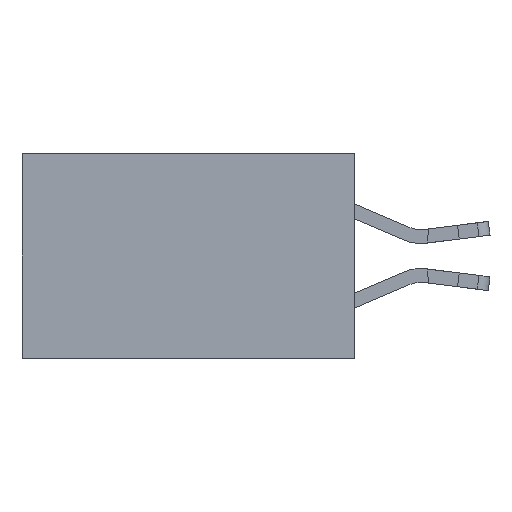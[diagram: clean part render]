
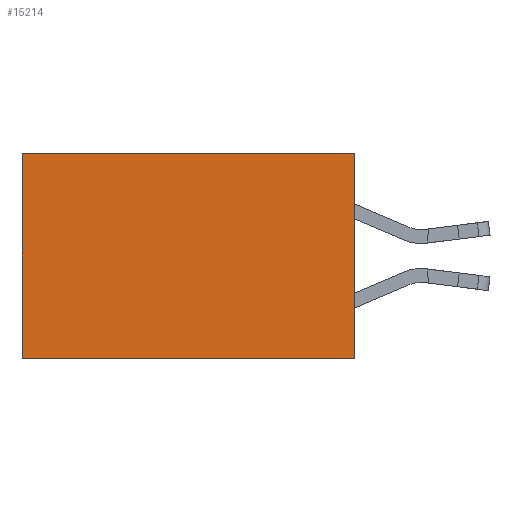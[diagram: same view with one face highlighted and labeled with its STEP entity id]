
A CAD part, left-side view. The second image highlights one B-rep face of the part: STEP entity #15214.
In plain terms, the highlighted planar face has unit normal (-1, 0, 0).
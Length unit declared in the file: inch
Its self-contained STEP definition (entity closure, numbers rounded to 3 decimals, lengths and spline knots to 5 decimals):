
#25 = CARTESIAN_POINT ( 'NONE',  ( 0.298, 0., 0. ) ) ;
#1028 = ORIENTED_EDGE ( 'NONE', *, *, #16419, .T. ) ;
#1622 = AXIS2_PLACEMENT_3D ( 'NONE', #9957, #19047, #8175 ) ;
#1727 = EDGE_CURVE ( 'NONE', #8493, #19266, #16690, .T. ) ;
#2264 = CARTESIAN_POINT ( 'NONE',  ( 0.298, 0.6, 0. ) ) ;
#2305 = CARTESIAN_POINT ( 'NONE',  ( 0.298, 0., -0.37 ) ) ;
#2420 = CARTESIAN_POINT ( 'NONE',  ( 0.298, 0., 0. ) ) ;
#2468 = PLANE ( 'NONE',  #1622 ) ;
#4187 = LINE ( 'NONE', #2420, #22851 ) ;
#4467 = DIRECTION ( 'NONE',  ( 0., 1., 0. ) ) ;
#8175 = DIRECTION ( 'NONE',  ( 0., 0., -1. ) ) ;
#8493 = VERTEX_POINT ( 'NONE', #21633 ) ;
#8758 = VERTEX_POINT ( 'NONE', #2305 ) ;
#9016 = LINE ( 'NONE', #18763, #22746 ) ;
#9944 = VECTOR ( 'NONE', #12776, 39.37008 ) ;
#9957 = CARTESIAN_POINT ( 'NONE',  ( 0.298, 0., 0. ) ) ;
#11670 = EDGE_CURVE ( 'NONE', #8493, #8758, #4187, .T. ) ;
#11804 = DIRECTION ( 'NONE',  ( 0., 0., -1. ) ) ;
#11878 = VECTOR ( 'NONE', #4467, 39.37008 ) ;
#12776 = DIRECTION ( 'NONE',  ( 0., 1., 0. ) ) ;
#14910 = EDGE_CURVE ( 'NONE', #8758, #15869, #19004, .T. ) ;
#15214 = ADVANCED_FACE ( 'NONE', ( #22249 ), #2468, .F. ) ;
#15481 = ORIENTED_EDGE ( 'NONE', *, *, #1727, .T. ) ;
#15865 = ORIENTED_EDGE ( 'NONE', *, *, #14910, .F. ) ;
#15869 = VERTEX_POINT ( 'NONE', #22524 ) ;
#16419 = EDGE_CURVE ( 'NONE', #19266, #15869, #9016, .T. ) ;
#16690 = LINE ( 'NONE', #25, #11878 ) ;
#17492 = ORIENTED_EDGE ( 'NONE', *, *, #11670, .F. ) ;
#18763 = CARTESIAN_POINT ( 'NONE',  ( 0.298, 0.6, 0. ) ) ;
#19004 = LINE ( 'NONE', #21599, #9944 ) ;
#19047 = DIRECTION ( 'NONE',  ( 1., 0., 0. ) ) ;
#19266 = VERTEX_POINT ( 'NONE', #2264 ) ;
#20534 = DIRECTION ( 'NONE',  ( 0., 0., -1. ) ) ;
#21599 = CARTESIAN_POINT ( 'NONE',  ( 0.298, 0., -0.37 ) ) ;
#21633 = CARTESIAN_POINT ( 'NONE',  ( 0.298, 0., 0. ) ) ;
#22063 = EDGE_LOOP ( 'NONE', ( #1028, #15865, #17492, #15481 ) ) ;
#22249 = FACE_OUTER_BOUND ( 'NONE', #22063, .T. ) ;
#22524 = CARTESIAN_POINT ( 'NONE',  ( 0.298, 0.6, -0.37 ) ) ;
#22746 = VECTOR ( 'NONE', #20534, 39.37008 ) ;
#22851 = VECTOR ( 'NONE', #11804, 39.37008 ) ;
